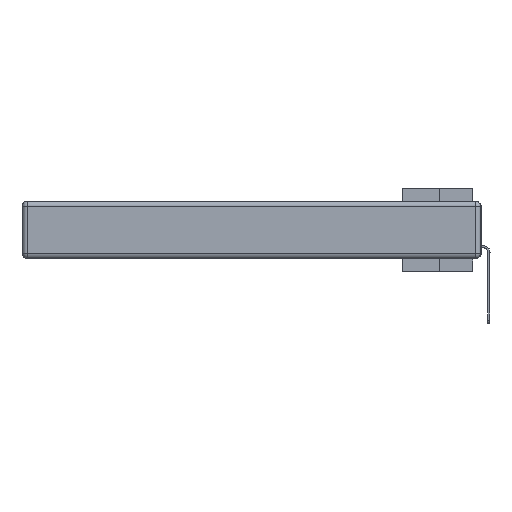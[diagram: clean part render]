
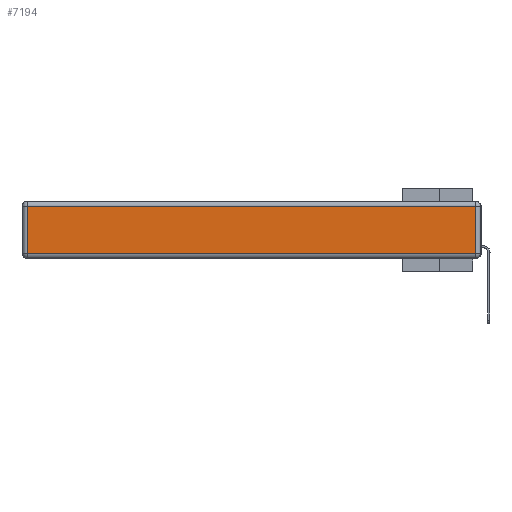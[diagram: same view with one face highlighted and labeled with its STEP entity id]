
A CAD part, left-side view. The second image highlights one B-rep face of the part: STEP entity #7194.
In plain terms, the highlighted planar face has unit normal (-1, 0, 0).
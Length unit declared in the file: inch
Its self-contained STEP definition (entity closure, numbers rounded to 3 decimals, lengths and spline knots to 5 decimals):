
#2689 = CARTESIAN_POINT ( 'NONE',  ( 0., 0., -0.343 ) ) ;
#3475 = DIRECTION ( 'NONE',  ( 0., 0., 1. ) ) ;
#3552 = ORIENTED_EDGE ( 'NONE', *, *, #22143, .T. ) ;
#4667 = VERTEX_POINT ( 'NONE', #9394 ) ;
#5064 = ORIENTED_EDGE ( 'NONE', *, *, #38062, .T. ) ;
#5143 = LINE ( 'NONE', #28727, #36002 ) ;
#7194 = ADVANCED_FACE ( 'NONE', ( #8607 ), #35728, .T. ) ;
#7540 = CARTESIAN_POINT ( 'NONE',  ( 0., 0., -0.313 ) ) ;
#7584 = CARTESIAN_POINT ( 'NONE',  ( 0., 2.72, -0.03 ) ) ;
#8447 = EDGE_CURVE ( 'NONE', #32065, #33439, #5143, .T. ) ;
#8607 = FACE_OUTER_BOUND ( 'NONE', #19396, .T. ) ;
#8759 = CARTESIAN_POINT ( 'NONE',  ( 0., 2.72, -0.343 ) ) ;
#8828 = EDGE_CURVE ( 'NONE', #33439, #4667, #26829, .T. ) ;
#9394 = CARTESIAN_POINT ( 'NONE',  ( 0., 2.72, -0.313 ) ) ;
#10077 = VERTEX_POINT ( 'NONE', #13490 ) ;
#12035 = ORIENTED_EDGE ( 'NONE', *, *, #8447, .T. ) ;
#13490 = CARTESIAN_POINT ( 'NONE',  ( 0., 0.03, -0.313 ) ) ;
#14057 = AXIS2_PLACEMENT_3D ( 'NONE', #2689, #38692, #32778 ) ;
#16521 = ORIENTED_EDGE ( 'NONE', *, *, #8828, .T. ) ;
#17037 = DIRECTION ( 'NONE',  ( 0., 0., -1. ) ) ;
#17834 = VECTOR ( 'NONE', #17037, 39.37008 ) ;
#19396 = EDGE_LOOP ( 'NONE', ( #3552, #5064, #12035, #16521 ) ) ;
#19543 = DIRECTION ( 'NONE',  ( 0., -1., 0. ) ) ;
#22143 = EDGE_CURVE ( 'NONE', #4667, #10077, #37416, .T. ) ;
#22633 = DIRECTION ( 'NONE',  ( 0., 1., 0. ) ) ;
#26829 = LINE ( 'NONE', #8759, #17834 ) ;
#28727 = CARTESIAN_POINT ( 'NONE',  ( 0., 2.75, -0.03 ) ) ;
#30640 = VECTOR ( 'NONE', #3475, 39.37008 ) ;
#30990 = LINE ( 'NONE', #33369, #30640 ) ;
#32065 = VERTEX_POINT ( 'NONE', #32946 ) ;
#32166 = VECTOR ( 'NONE', #19543, 39.37008 ) ;
#32778 = DIRECTION ( 'NONE',  ( 0., 0., 1. ) ) ;
#32946 = CARTESIAN_POINT ( 'NONE',  ( 0., 0.03, -0.03 ) ) ;
#33369 = CARTESIAN_POINT ( 'NONE',  ( 0., 0.03, -0.343 ) ) ;
#33439 = VERTEX_POINT ( 'NONE', #7584 ) ;
#35728 = PLANE ( 'NONE',  #14057 ) ;
#36002 = VECTOR ( 'NONE', #22633, 39.37008 ) ;
#37416 = LINE ( 'NONE', #7540, #32166 ) ;
#38062 = EDGE_CURVE ( 'NONE', #10077, #32065, #30990, .T. ) ;
#38692 = DIRECTION ( 'NONE',  ( -1., 0., 0. ) ) ;
